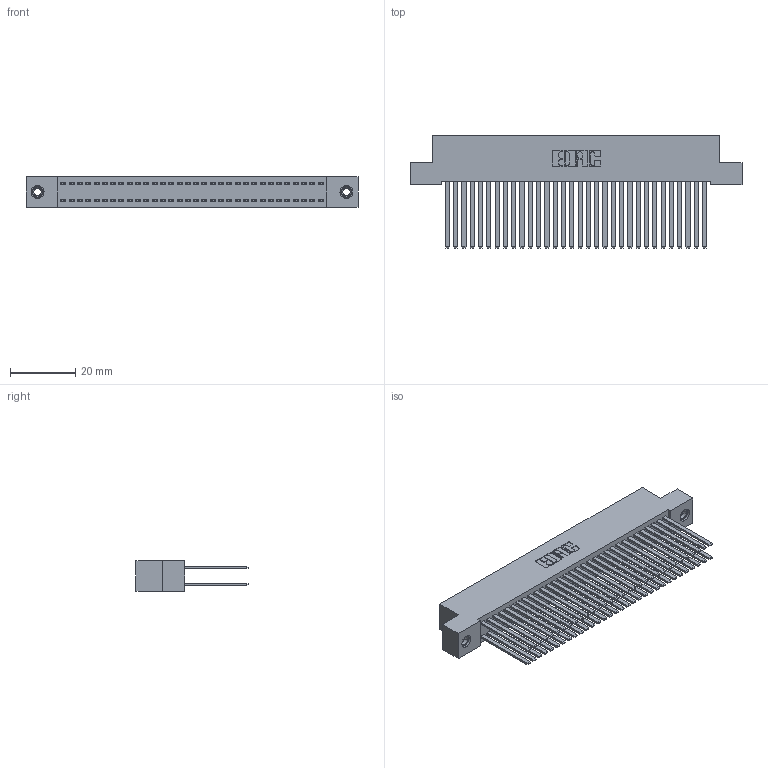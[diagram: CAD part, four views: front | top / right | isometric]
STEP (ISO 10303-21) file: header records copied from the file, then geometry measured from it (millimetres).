
FILE_DESCRIPTION (( 'STEP AP203' ), '1' );
FILE_NAME ('342-064-544-208.STEP', '2019-10-03T14:29:59', ( '' ), ( '' ), 'SwSTEP 2.0', 'SolidWorks 2016', '' );
FILE_SCHEMA (( 'CONFIG_CONTROL_DESIGN' ));
Length unit declared in the file: inch
Products named in the file (4): 342 Part_TI; 345-292-001_345-293-144; 345-250-001_345-250-003-102; 342-064-544-208
Assembly tree (67 placements, depth 2):
  342-064-544-208
    342 Part_TI
    345-292-001_345-293-144  x64
    345-250-001_345-250-003-102  x2
Bounding box: 101.6 x 34.3 x 9.4 mm (x, y, z)
Volume: 9972.9 mm3; surface area: 18481.8 mm2
Topology: 67 solids, 67 shells, 3114 faces, 9203 edges, 6042 vertices
Faces by surface type: plane 2146, cylinder 952, cone 12, torus 4
Entity records: 22750 total; most frequent: CARTESIAN_POINT 3761, ORIENTED_EDGE 3690, DIRECTION 3259, EDGE_CURVE 1845, VECTOR 1701, LINE 1701, VERTEX_POINT 1224, AXIS2_PLACEMENT_3D 779
